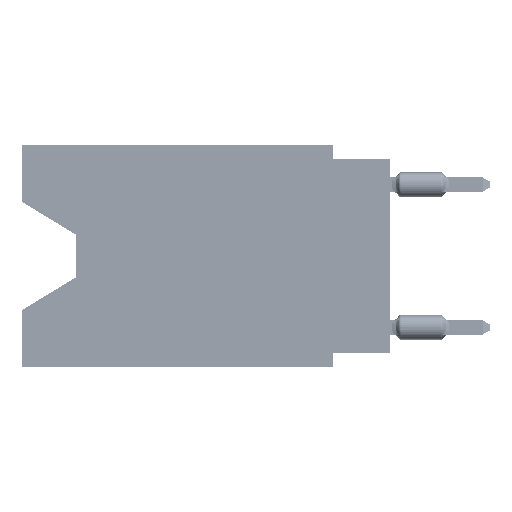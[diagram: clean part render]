
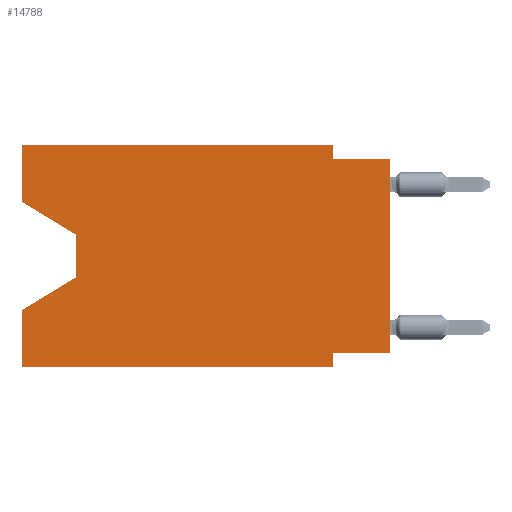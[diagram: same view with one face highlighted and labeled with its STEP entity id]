
A CAD part, left-side view. The second image highlights one B-rep face of the part: STEP entity #14788.
In plain terms, the highlighted planar face has unit normal (-1, 0, 0).
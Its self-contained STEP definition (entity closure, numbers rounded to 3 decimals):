
#447 = VERTEX_POINT ( 'NONE', #31926 ) ;
#1255 = VERTEX_POINT ( 'NONE', #68525 ) ;
#1544 = CARTESIAN_POINT ( 'NONE',  ( 0., 2.54, -9.906 ) ) ;
#2070 = EDGE_CURVE ( 'NONE', #66131, #27045, #74240, .T. ) ;
#2758 = DIRECTION ( 'NONE',  ( 0., 0., 1. ) ) ;
#2989 = VERTEX_POINT ( 'NONE', #7813 ) ;
#3520 = CARTESIAN_POINT ( 'NONE',  ( 0., 2.54, 0. ) ) ;
#5564 = ORIENTED_EDGE ( 'NONE', *, *, #14789, .T. ) ;
#7417 = LINE ( 'NONE', #1544, #27465 ) ;
#7813 = CARTESIAN_POINT ( 'NONE',  ( 0., 0., -9.271 ) ) ;
#8995 = EDGE_CURVE ( 'NONE', #71185, #46408, #52848, .T. ) ;
#11561 = VECTOR ( 'NONE', #73534, 1000. ) ;
#12648 = CARTESIAN_POINT ( 'NONE',  ( 0., 16.383, 0. ) ) ;
#13714 = DIRECTION ( 'NONE',  ( 0., 0., -1. ) ) ;
#14788 = ADVANCED_FACE ( 'NONE', ( #76744 ), #64945, .F. ) ;
#14789 = EDGE_CURVE ( 'NONE', #47445, #447, #31476, .T. ) ;
#16752 = ORIENTED_EDGE ( 'NONE', *, *, #64299, .F. ) ;
#18051 = CARTESIAN_POINT ( 'NONE',  ( 0., 16.383, 0. ) ) ;
#18213 = VECTOR ( 'NONE', #25275, 1000. ) ;
#18533 = DIRECTION ( 'NONE',  ( 0., 0., -1. ) ) ;
#21381 = VERTEX_POINT ( 'NONE', #63762 ) ;
#21566 = AXIS2_PLACEMENT_3D ( 'NONE', #12648, #53945, #18533 ) ;
#22958 = EDGE_CURVE ( 'NONE', #2989, #21381, #35885, .T. ) ;
#23240 = CARTESIAN_POINT ( 'NONE',  ( 0., 13.97, -4.013 ) ) ;
#23408 = VECTOR ( 'NONE', #65683, 1000. ) ;
#23454 = EDGE_CURVE ( 'NONE', #447, #66131, #77082, .T. ) ;
#24949 = EDGE_CURVE ( 'NONE', #46408, #34151, #45575, .T. ) ;
#25275 = DIRECTION ( 'NONE',  ( 0., -1., 0. ) ) ;
#25373 = CARTESIAN_POINT ( 'NONE',  ( 0., 16.383, 0. ) ) ;
#27045 = VERTEX_POINT ( 'NONE', #75941 ) ;
#27465 = VECTOR ( 'NONE', #13714, 1000. ) ;
#28540 = ORIENTED_EDGE ( 'NONE', *, *, #8995, .F. ) ;
#29016 = CARTESIAN_POINT ( 'NONE',  ( 0., 16.383, -9.906 ) ) ;
#29632 = VECTOR ( 'NONE', #59854, 1000. ) ;
#31476 = LINE ( 'NONE', #73153, #11561 ) ;
#31662 = DIRECTION ( 'NONE',  ( 0., 0., 1. ) ) ;
#31926 = CARTESIAN_POINT ( 'NONE',  ( 0., 13.97, -4.013 ) ) ;
#33542 = VECTOR ( 'NONE', #75432, 1000. ) ;
#33880 = VECTOR ( 'NONE', #2758, 1000. ) ;
#34151 = VERTEX_POINT ( 'NONE', #76010 ) ;
#35885 = LINE ( 'NONE', #70886, #29632 ) ;
#37805 = ORIENTED_EDGE ( 'NONE', *, *, #38896, .T. ) ;
#38896 = EDGE_CURVE ( 'NONE', #2989, #1255, #39292, .T. ) ;
#39292 = LINE ( 'NONE', #74664, #33880 ) ;
#39949 = VERTEX_POINT ( 'NONE', #70534 ) ;
#40550 = ORIENTED_EDGE ( 'NONE', *, *, #2070, .T. ) ;
#40693 = ORIENTED_EDGE ( 'NONE', *, *, #24949, .F. ) ;
#43453 = LINE ( 'NONE', #25373, #48998 ) ;
#43783 = EDGE_LOOP ( 'NONE', ( #5564, #45131, #40550, #16752, #45283, #46329, #59048, #37805, #71666, #40693, #28540, #58573 ) ) ;
#44375 = CARTESIAN_POINT ( 'NONE',  ( 0., 16.383, -2.546 ) ) ;
#45131 = ORIENTED_EDGE ( 'NONE', *, *, #23454, .T. ) ;
#45283 = ORIENTED_EDGE ( 'NONE', *, *, #69327, .T. ) ;
#45575 = LINE ( 'NONE', #3520, #33542 ) ;
#46329 = ORIENTED_EDGE ( 'NONE', *, *, #60780, .F. ) ;
#46408 = VERTEX_POINT ( 'NONE', #54418 ) ;
#46955 = DIRECTION ( 'NONE',  ( 0., -1., 0. ) ) ;
#47445 = VERTEX_POINT ( 'NONE', #44375 ) ;
#48111 = CARTESIAN_POINT ( 'NONE',  ( 0., 0., -0.635 ) ) ;
#48998 = VECTOR ( 'NONE', #31662, 1000. ) ;
#49481 = CARTESIAN_POINT ( 'NONE',  ( 0., 13.97, -5.893 ) ) ;
#51070 = VECTOR ( 'NONE', #46955, 1000. ) ;
#52756 = LINE ( 'NONE', #18051, #58329 ) ;
#52848 = LINE ( 'NONE', #76812, #51070 ) ;
#53945 = DIRECTION ( 'NONE',  ( 1., 0., 0. ) ) ;
#54014 = LINE ( 'NONE', #48111, #18213 ) ;
#54418 = CARTESIAN_POINT ( 'NONE',  ( 0., 2.54, 0. ) ) ;
#55620 = VECTOR ( 'NONE', #76570, 1000. ) ;
#55979 = EDGE_CURVE ( 'NONE', #47445, #71185, #52756, .T. ) ;
#56819 = VECTOR ( 'NONE', #60511, 1000. ) ;
#56875 = EDGE_CURVE ( 'NONE', #34151, #1255, #54014, .T. ) ;
#58329 = VECTOR ( 'NONE', #70442, 1000. ) ;
#58573 = ORIENTED_EDGE ( 'NONE', *, *, #55979, .F. ) ;
#59048 = ORIENTED_EDGE ( 'NONE', *, *, #22958, .F. ) ;
#59854 = DIRECTION ( 'NONE',  ( 0., 1., 0. ) ) ;
#60511 = DIRECTION ( 'NONE',  ( 0., 0.855, -0.519 ) ) ;
#60780 = EDGE_CURVE ( 'NONE', #21381, #66296, #7417, .T. ) ;
#63762 = CARTESIAN_POINT ( 'NONE',  ( 0., 2.54, -9.271 ) ) ;
#64299 = EDGE_CURVE ( 'NONE', #39949, #27045, #43453, .T. ) ;
#64945 = PLANE ( 'NONE',  #21566 ) ;
#65683 = DIRECTION ( 'NONE',  ( 0., 0., -1. ) ) ;
#66131 = VERTEX_POINT ( 'NONE', #74205 ) ;
#66296 = VERTEX_POINT ( 'NONE', #69867 ) ;
#68525 = CARTESIAN_POINT ( 'NONE',  ( 0., 0., -0.635 ) ) ;
#69327 = EDGE_CURVE ( 'NONE', #39949, #66296, #72217, .T. ) ;
#69867 = CARTESIAN_POINT ( 'NONE',  ( 0., 2.54, -9.906 ) ) ;
#70442 = DIRECTION ( 'NONE',  ( 0., 0., 1. ) ) ;
#70534 = CARTESIAN_POINT ( 'NONE',  ( 0., 16.383, -9.906 ) ) ;
#70886 = CARTESIAN_POINT ( 'NONE',  ( 0., 0., -9.271 ) ) ;
#71185 = VERTEX_POINT ( 'NONE', #72172 ) ;
#71666 = ORIENTED_EDGE ( 'NONE', *, *, #56875, .F. ) ;
#72172 = CARTESIAN_POINT ( 'NONE',  ( 0., 16.383, 0. ) ) ;
#72217 = LINE ( 'NONE', #29016, #55620 ) ;
#73153 = CARTESIAN_POINT ( 'NONE',  ( 0., 16.383, -2.546 ) ) ;
#73534 = DIRECTION ( 'NONE',  ( 0., -0.855, -0.519 ) ) ;
#74205 = CARTESIAN_POINT ( 'NONE',  ( 0., 13.97, -5.893 ) ) ;
#74240 = LINE ( 'NONE', #49481, #56819 ) ;
#74664 = CARTESIAN_POINT ( 'NONE',  ( 0., 0., 0. ) ) ;
#75432 = DIRECTION ( 'NONE',  ( 0., 0., -1. ) ) ;
#75941 = CARTESIAN_POINT ( 'NONE',  ( 0., 16.383, -7.36 ) ) ;
#76010 = CARTESIAN_POINT ( 'NONE',  ( 0., 2.54, -0.635 ) ) ;
#76570 = DIRECTION ( 'NONE',  ( 0., -1., 0. ) ) ;
#76744 = FACE_OUTER_BOUND ( 'NONE', #43783, .T. ) ;
#76812 = CARTESIAN_POINT ( 'NONE',  ( 0., 16.383, 0. ) ) ;
#77082 = LINE ( 'NONE', #23240, #23408 ) ;
